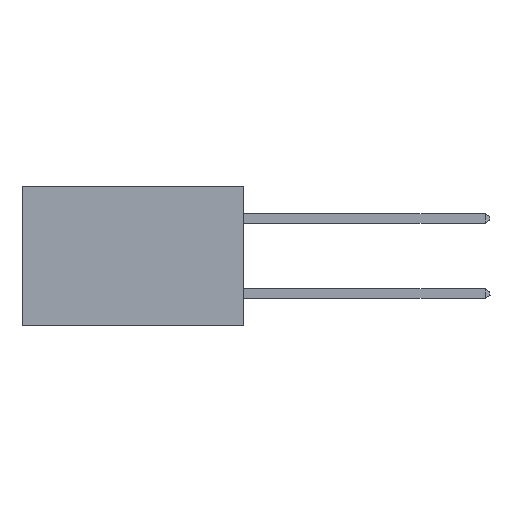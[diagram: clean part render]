
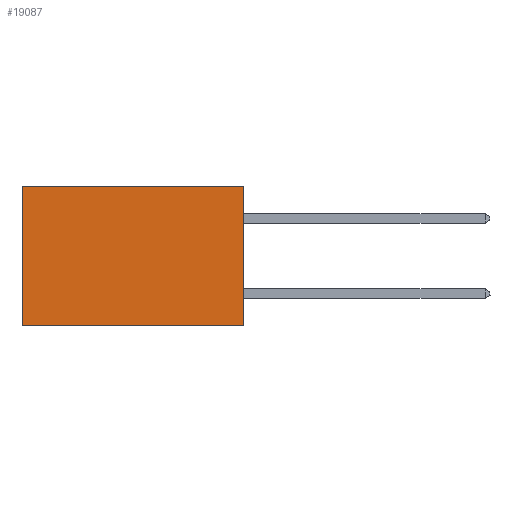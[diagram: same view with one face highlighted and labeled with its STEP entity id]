
A CAD part, left-side view. The second image highlights one B-rep face of the part: STEP entity #19087.
In plain terms, the highlighted planar face has unit normal (-1, 0, 0).
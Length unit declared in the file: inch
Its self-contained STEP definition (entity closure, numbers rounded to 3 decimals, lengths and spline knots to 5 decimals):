
#2217 = CARTESIAN_POINT ( 'NONE',  ( 0.277, 0., -0.37 ) ) ;
#2832 = PLANE ( 'NONE',  #11325 ) ;
#2903 = CARTESIAN_POINT ( 'NONE',  ( 0.277, 0., -0.37 ) ) ;
#2984 = DIRECTION ( 'NONE',  ( 0., 1., 0. ) ) ;
#3069 = VERTEX_POINT ( 'NONE', #8293 ) ;
#3673 = LINE ( 'NONE', #2903, #12071 ) ;
#3926 = CARTESIAN_POINT ( 'NONE',  ( 0.277, 0., -0.37 ) ) ;
#4608 = DIRECTION ( 'NONE',  ( 0., 0., -1. ) ) ;
#4952 = VERTEX_POINT ( 'NONE', #8504 ) ;
#5333 = LINE ( 'NONE', #2217, #18443 ) ;
#5585 = DIRECTION ( 'NONE',  ( 0., 0., -1. ) ) ;
#5737 = EDGE_CURVE ( 'NONE', #8912, #4952, #11811, .T. ) ;
#5971 = EDGE_CURVE ( 'NONE', #3069, #8912, #15695, .T. ) ;
#6364 = ORIENTED_EDGE ( 'NONE', *, *, #22013, .F. ) ;
#6418 = CARTESIAN_POINT ( 'NONE',  ( 0.277, 0.59, -0.37 ) ) ;
#7010 = EDGE_LOOP ( 'NONE', ( #21165, #6364, #20969, #11808 ) ) ;
#8293 = CARTESIAN_POINT ( 'NONE',  ( 0.277, 0., 0. ) ) ;
#8504 = CARTESIAN_POINT ( 'NONE',  ( 0.277, 0.59, -0.37 ) ) ;
#8912 = VERTEX_POINT ( 'NONE', #14455 ) ;
#9302 = DIRECTION ( 'NONE',  ( 0., 0., -1. ) ) ;
#10390 = VERTEX_POINT ( 'NONE', #3926 ) ;
#10961 = VECTOR ( 'NONE', #19663, 39.37008 ) ;
#11325 = AXIS2_PLACEMENT_3D ( 'NONE', #22339, #15313, #4608 ) ;
#11808 = ORIENTED_EDGE ( 'NONE', *, *, #5971, .T. ) ;
#11811 = LINE ( 'NONE', #6418, #20690 ) ;
#12071 = VECTOR ( 'NONE', #2984, 39.37008 ) ;
#13478 = FACE_OUTER_BOUND ( 'NONE', #7010, .T. ) ;
#14455 = CARTESIAN_POINT ( 'NONE',  ( 0.277, 0.59, 0. ) ) ;
#15313 = DIRECTION ( 'NONE',  ( 1., 0., 0. ) ) ;
#15695 = LINE ( 'NONE', #20485, #10961 ) ;
#18443 = VECTOR ( 'NONE', #9302, 39.37008 ) ;
#18854 = EDGE_CURVE ( 'NONE', #3069, #10390, #5333, .T. ) ;
#19087 = ADVANCED_FACE ( 'NONE', ( #13478 ), #2832, .F. ) ;
#19663 = DIRECTION ( 'NONE',  ( 0., 1., 0. ) ) ;
#20485 = CARTESIAN_POINT ( 'NONE',  ( 0.277, 0., 0. ) ) ;
#20690 = VECTOR ( 'NONE', #5585, 39.37008 ) ;
#20969 = ORIENTED_EDGE ( 'NONE', *, *, #18854, .F. ) ;
#21165 = ORIENTED_EDGE ( 'NONE', *, *, #5737, .T. ) ;
#22013 = EDGE_CURVE ( 'NONE', #10390, #4952, #3673, .T. ) ;
#22339 = CARTESIAN_POINT ( 'NONE',  ( 0.277, 0., -0.37 ) ) ;
